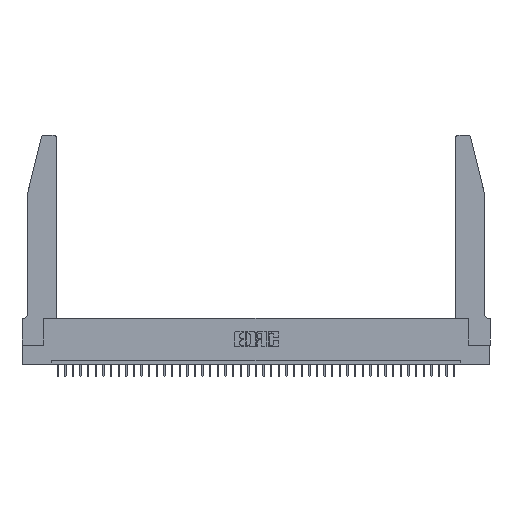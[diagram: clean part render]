
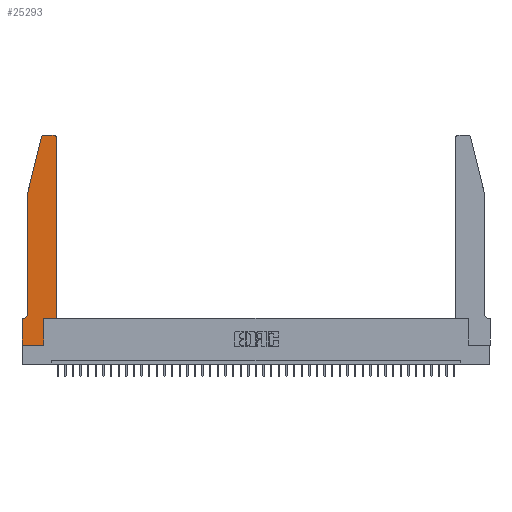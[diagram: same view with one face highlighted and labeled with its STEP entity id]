
A CAD part, top view. The second image highlights one B-rep face of the part: STEP entity #25293.
In plain terms, the highlighted planar face has unit normal (0, 0, 1).
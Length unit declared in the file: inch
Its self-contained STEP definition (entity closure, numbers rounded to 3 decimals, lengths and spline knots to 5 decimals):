
#94 = VECTOR ( 'NONE', #17986, 39.37008 ) ;
#1127 = LINE ( 'NONE', #1355, #37141 ) ;
#1355 = CARTESIAN_POINT ( 'NONE',  ( 0.4505, 0.35, 0.37 ) ) ;
#1650 = DIRECTION ( 'NONE',  ( 1., 0., 0. ) ) ;
#2019 = DIRECTION ( 'NONE',  ( 1., 0., 0. ) ) ;
#2657 = CARTESIAN_POINT ( 'NONE',  ( 0.0755, 0.35, 0.37 ) ) ;
#3341 = VERTEX_POINT ( 'NONE', #20836 ) ;
#4658 = DIRECTION ( 'NONE',  ( 1., 0., 0. ) ) ;
#5602 = DIRECTION ( 'NONE',  ( -1., 0., 0. ) ) ;
#5749 = DIRECTION ( 'NONE',  ( -1., 0., 0. ) ) ;
#6819 = EDGE_CURVE ( 'NONE', #19961, #29731, #1127, .T. ) ;
#7439 = CARTESIAN_POINT ( 'NONE',  ( 0.4505, 0.35, 0.37 ) ) ;
#7457 = CARTESIAN_POINT ( 'NONE',  ( 0.25487, 2.72718, 0.37 ) ) ;
#7565 = CARTESIAN_POINT ( 'NONE',  ( 0.284, 2.72, 0.37 ) ) ;
#8099 = DIRECTION ( 'NONE',  ( -0.239, -0.971, 0. ) ) ;
#8954 = CIRCLE ( 'NONE', #36692, 0.03 ) ;
#9788 = LINE ( 'NONE', #39310, #20245 ) ;
#9835 = LINE ( 'NONE', #25700, #10325 ) ;
#10325 = VECTOR ( 'NONE', #15594, 39.37008 ) ;
#10665 = ORIENTED_EDGE ( 'NONE', *, *, #14649, .T. ) ;
#10746 = CARTESIAN_POINT ( 'NONE',  ( 0.4205, 2.75, 0.37 ) ) ;
#11532 = ORIENTED_EDGE ( 'NONE', *, *, #6819, .T. ) ;
#11862 = VERTEX_POINT ( 'NONE', #7457 ) ;
#12284 = DIRECTION ( 'NONE',  ( 0., 0., -1. ) ) ;
#13026 = EDGE_CURVE ( 'NONE', #30475, #11862, #24796, .T. ) ;
#13799 = ORIENTED_EDGE ( 'NONE', *, *, #22623, .T. ) ;
#14649 = EDGE_CURVE ( 'NONE', #27389, #39928, #8954, .T. ) ;
#15429 = LINE ( 'NONE', #23906, #38907 ) ;
#15555 = CARTESIAN_POINT ( 'NONE',  ( 0., 0.35, 0.37 ) ) ;
#15594 = DIRECTION ( 'NONE',  ( 0., -1., 0. ) ) ;
#15609 = ORIENTED_EDGE ( 'NONE', *, *, #39865, .T. ) ;
#16136 = DIRECTION ( 'NONE',  ( 1., 0., 0. ) ) ;
#16230 = AXIS2_PLACEMENT_3D ( 'NONE', #15555, #22447, #2019 ) ;
#17086 = CARTESIAN_POINT ( 'NONE',  ( 0.4505, 2.72, 0.37 ) ) ;
#17848 = EDGE_CURVE ( 'NONE', #29758, #27288, #9788, .T. ) ;
#17986 = DIRECTION ( 'NONE',  ( 0., -1., 0. ) ) ;
#18749 = LINE ( 'NONE', #34349, #31257 ) ;
#18807 = EDGE_CURVE ( 'NONE', #29557, #29758, #9835, .T. ) ;
#19748 = ORIENTED_EDGE ( 'NONE', *, *, #18807, .T. ) ;
#19961 = VERTEX_POINT ( 'NONE', #37962 ) ;
#20026 = DIRECTION ( 'NONE',  ( 1., 0., 0. ) ) ;
#20245 = VECTOR ( 'NONE', #16136, 39.37008 ) ;
#20833 = DIRECTION ( 'NONE',  ( 0., 1., 0. ) ) ;
#20836 = CARTESIAN_POINT ( 'NONE',  ( 0.0755, 0.42, 0.37 ) ) ;
#20858 = EDGE_CURVE ( 'NONE', #11862, #23061, #15429, .T. ) ;
#20995 = DIRECTION ( 'NONE',  ( 0., 0., 1. ) ) ;
#21144 = EDGE_LOOP ( 'NONE', ( #40282, #34203, #31323, #29321, #31256, #28833, #19748, #27717, #15609, #11532, #13799, #10665 ) ) ;
#21506 = LINE ( 'NONE', #40693, #42435 ) ;
#22097 = VERTEX_POINT ( 'NONE', #37757 ) ;
#22387 = CARTESIAN_POINT ( 'NONE',  ( 0.0055, 0.42, 0.37 ) ) ;
#22447 = DIRECTION ( 'NONE',  ( 0., 0., 1. ) ) ;
#22623 = EDGE_CURVE ( 'NONE', #29731, #27389, #21506, .T. ) ;
#23061 = VERTEX_POINT ( 'NONE', #39490 ) ;
#23109 = FACE_OUTER_BOUND ( 'NONE', #21144, .T. ) ;
#23906 = CARTESIAN_POINT ( 'NONE',  ( 0.0755, 2., 0.37 ) ) ;
#24115 = VECTOR ( 'NONE', #5749, 39.37008 ) ;
#24729 = CARTESIAN_POINT ( 'NONE',  ( 0.0755, 2., 0.37 ) ) ;
#24796 = CIRCLE ( 'NONE', #28038, 0.03 ) ;
#24847 = EDGE_CURVE ( 'NONE', #22097, #29557, #41935, .T. ) ;
#25112 = LINE ( 'NONE', #24729, #94 ) ;
#25293 = ADVANCED_FACE ( 'NONE', ( #23109 ), #35522, .T. ) ;
#25646 = EDGE_CURVE ( 'NONE', #23061, #3341, #25112, .T. ) ;
#25700 = CARTESIAN_POINT ( 'NONE',  ( 0., 0., 0.37 ) ) ;
#25742 = CARTESIAN_POINT ( 'NONE',  ( 0.2605, 2.75, 0.37 ) ) ;
#26011 = DIRECTION ( 'NONE',  ( -1., 0., 0. ) ) ;
#26793 = CIRCLE ( 'NONE', #32860, 0.07 ) ;
#27288 = VERTEX_POINT ( 'NONE', #29961 ) ;
#27389 = VERTEX_POINT ( 'NONE', #17086 ) ;
#27717 = ORIENTED_EDGE ( 'NONE', *, *, #17848, .T. ) ;
#28038 = AXIS2_PLACEMENT_3D ( 'NONE', #7565, #20995, #4658 ) ;
#28833 = ORIENTED_EDGE ( 'NONE', *, *, #24847, .T. ) ;
#29321 = ORIENTED_EDGE ( 'NONE', *, *, #25646, .T. ) ;
#29557 = VERTEX_POINT ( 'NONE', #36049 ) ;
#29731 = VERTEX_POINT ( 'NONE', #7439 ) ;
#29758 = VERTEX_POINT ( 'NONE', #40725 ) ;
#29961 = CARTESIAN_POINT ( 'NONE',  ( 0.2865, 0., 0.37 ) ) ;
#30475 = VERTEX_POINT ( 'NONE', #37143 ) ;
#30599 = DIRECTION ( 'NONE',  ( 0., 1., 0. ) ) ;
#31256 = ORIENTED_EDGE ( 'NONE', *, *, #40743, .T. ) ;
#31257 = VECTOR ( 'NONE', #30599, 39.37008 ) ;
#31323 = ORIENTED_EDGE ( 'NONE', *, *, #20858, .T. ) ;
#32860 = AXIS2_PLACEMENT_3D ( 'NONE', #22387, #12284, #5602 ) ;
#34189 = CARTESIAN_POINT ( 'NONE',  ( 0.4205, 2.72, 0.37 ) ) ;
#34203 = ORIENTED_EDGE ( 'NONE', *, *, #13026, .T. ) ;
#34349 = CARTESIAN_POINT ( 'NONE',  ( 0.2865, 0.35, 0.37 ) ) ;
#34467 = DIRECTION ( 'NONE',  ( 0., 0., 1. ) ) ;
#35522 = PLANE ( 'NONE',  #16230 ) ;
#36049 = CARTESIAN_POINT ( 'NONE',  ( 0., 0.35, 0.37 ) ) ;
#36692 = AXIS2_PLACEMENT_3D ( 'NONE', #34189, #34467, #20026 ) ;
#37141 = VECTOR ( 'NONE', #1650, 39.37008 ) ;
#37143 = CARTESIAN_POINT ( 'NONE',  ( 0.284, 2.75, 0.37 ) ) ;
#37159 = LINE ( 'NONE', #25742, #24115 ) ;
#37757 = CARTESIAN_POINT ( 'NONE',  ( 0.0055, 0.35, 0.37 ) ) ;
#37962 = CARTESIAN_POINT ( 'NONE',  ( 0.2865, 0.35, 0.37 ) ) ;
#38907 = VECTOR ( 'NONE', #8099, 39.37008 ) ;
#39310 = CARTESIAN_POINT ( 'NONE',  ( 0., 0., 0.37 ) ) ;
#39490 = CARTESIAN_POINT ( 'NONE',  ( 0.0755, 2., 0.37 ) ) ;
#39865 = EDGE_CURVE ( 'NONE', #27288, #19961, #18749, .T. ) ;
#39928 = VERTEX_POINT ( 'NONE', #10746 ) ;
#40282 = ORIENTED_EDGE ( 'NONE', *, *, #40757, .T. ) ;
#40693 = CARTESIAN_POINT ( 'NONE',  ( 0.4505, 0.35, 0.37 ) ) ;
#40725 = CARTESIAN_POINT ( 'NONE',  ( 0., 0., 0.37 ) ) ;
#40743 = EDGE_CURVE ( 'NONE', #3341, #22097, #26793, .T. ) ;
#40757 = EDGE_CURVE ( 'NONE', #39928, #30475, #37159, .T. ) ;
#40879 = VECTOR ( 'NONE', #26011, 39.37008 ) ;
#41935 = LINE ( 'NONE', #2657, #40879 ) ;
#42435 = VECTOR ( 'NONE', #20833, 39.37008 ) ;
